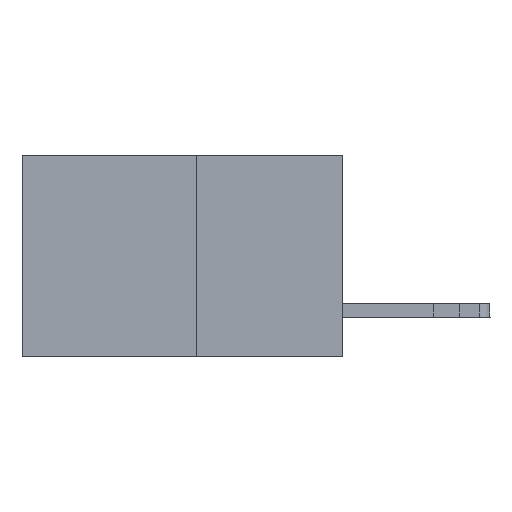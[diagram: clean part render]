
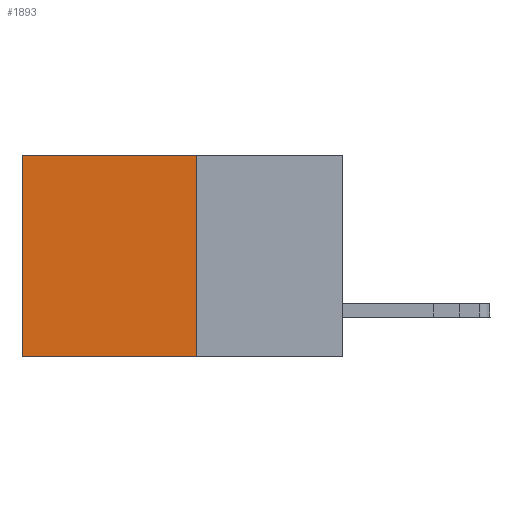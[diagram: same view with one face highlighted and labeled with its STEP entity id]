
A CAD part, left-side view. The second image highlights one B-rep face of the part: STEP entity #1893.
In plain terms, the highlighted planar face has unit normal (-1, 0, 0).
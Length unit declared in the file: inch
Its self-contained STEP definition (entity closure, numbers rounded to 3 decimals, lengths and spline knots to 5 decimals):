
#523 = CARTESIAN_POINT ( 'NONE',  ( 0.277, 0.27, -0.37 ) ) ;
#1656 = CARTESIAN_POINT ( 'NONE',  ( 0.277, 0.59, -0.37 ) ) ;
#1893 = ADVANCED_FACE ( 'NONE', ( #11682 ), #2827, .F. ) ;
#2076 = VECTOR ( 'NONE', #4312, 39.37008 ) ;
#2827 = PLANE ( 'NONE',  #5429 ) ;
#3910 = VECTOR ( 'NONE', #10644, 39.37008 ) ;
#3935 = VECTOR ( 'NONE', #12788, 39.37008 ) ;
#4102 = ORIENTED_EDGE ( 'NONE', *, *, #10581, .T. ) ;
#4217 = VERTEX_POINT ( 'NONE', #12386 ) ;
#4312 = DIRECTION ( 'NONE',  ( 0., 0., -1. ) ) ;
#4597 = EDGE_CURVE ( 'NONE', #4217, #10149, #12597, .T. ) ;
#4850 = CARTESIAN_POINT ( 'NONE',  ( 0.277, 0.59, 0. ) ) ;
#5002 = CARTESIAN_POINT ( 'NONE',  ( 0.277, 0.27, 0. ) ) ;
#5429 = AXIS2_PLACEMENT_3D ( 'NONE', #523, #11750, #11619 ) ;
#5465 = CARTESIAN_POINT ( 'NONE',  ( 0.277, 0.59, -0.37 ) ) ;
#5679 = VERTEX_POINT ( 'NONE', #11557 ) ;
#5865 = ORIENTED_EDGE ( 'NONE', *, *, #4597, .F. ) ;
#6414 = LINE ( 'NONE', #8378, #2076 ) ;
#6507 = EDGE_CURVE ( 'NONE', #5679, #4217, #6414, .T. ) ;
#7031 = LINE ( 'NONE', #5002, #7157 ) ;
#7157 = VECTOR ( 'NONE', #9118, 39.37008 ) ;
#7559 = LINE ( 'NONE', #5465, #3910 ) ;
#7702 = ORIENTED_EDGE ( 'NONE', *, *, #6507, .F. ) ;
#8378 = CARTESIAN_POINT ( 'NONE',  ( 0.277, 0.27, -0.37 ) ) ;
#9118 = DIRECTION ( 'NONE',  ( 0., 1., 0. ) ) ;
#9770 = CARTESIAN_POINT ( 'NONE',  ( 0.277, 0.27, -0.37 ) ) ;
#10149 = VERTEX_POINT ( 'NONE', #1656 ) ;
#10581 = EDGE_CURVE ( 'NONE', #12759, #10149, #7559, .T. ) ;
#10644 = DIRECTION ( 'NONE',  ( 0., 0., -1. ) ) ;
#11150 = ORIENTED_EDGE ( 'NONE', *, *, #12513, .T. ) ;
#11324 = EDGE_LOOP ( 'NONE', ( #4102, #5865, #7702, #11150 ) ) ;
#11557 = CARTESIAN_POINT ( 'NONE',  ( 0.277, 0.27, 0. ) ) ;
#11619 = DIRECTION ( 'NONE',  ( 0., 0., -1. ) ) ;
#11682 = FACE_OUTER_BOUND ( 'NONE', #11324, .T. ) ;
#11750 = DIRECTION ( 'NONE',  ( 1., 0., 0. ) ) ;
#12386 = CARTESIAN_POINT ( 'NONE',  ( 0.277, 0.27, -0.37 ) ) ;
#12513 = EDGE_CURVE ( 'NONE', #5679, #12759, #7031, .T. ) ;
#12597 = LINE ( 'NONE', #9770, #3935 ) ;
#12759 = VERTEX_POINT ( 'NONE', #4850 ) ;
#12788 = DIRECTION ( 'NONE',  ( 0., 1., 0. ) ) ;
